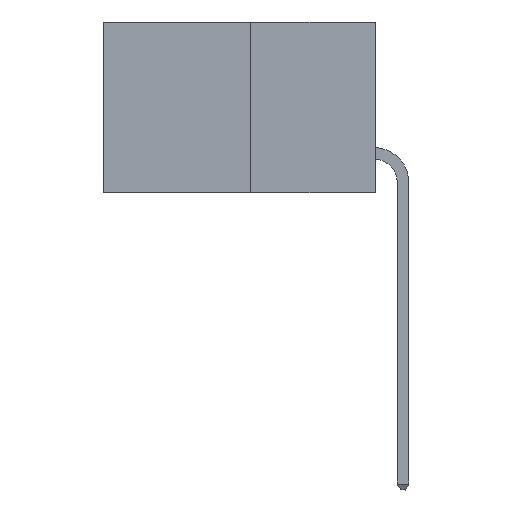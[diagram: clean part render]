
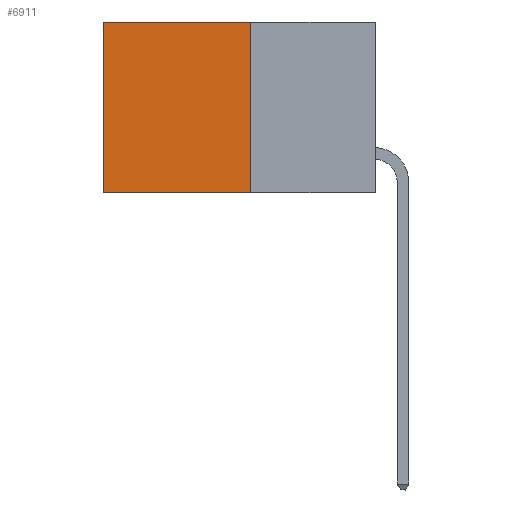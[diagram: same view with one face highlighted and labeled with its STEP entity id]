
A CAD part, left-side view. The second image highlights one B-rep face of the part: STEP entity #6911.
In plain terms, the highlighted planar face has unit normal (-1, 0, 0).
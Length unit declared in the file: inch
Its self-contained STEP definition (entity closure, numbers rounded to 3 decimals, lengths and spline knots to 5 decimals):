
#1206 = VECTOR ( 'NONE', #10832, 39.37008 ) ;
#1775 = VECTOR ( 'NONE', #4129, 39.37008 ) ;
#2823 = LINE ( 'NONE', #6025, #8602 ) ;
#3400 = DIRECTION ( 'NONE',  ( 0., 0., -1. ) ) ;
#4114 = CARTESIAN_POINT ( 'NONE',  ( 0.277, 0.27, 0. ) ) ;
#4129 = DIRECTION ( 'NONE',  ( 0., 1., 0. ) ) ;
#5355 = LINE ( 'NONE', #4114, #1775 ) ;
#5723 = VERTEX_POINT ( 'NONE', #5789 ) ;
#5789 = CARTESIAN_POINT ( 'NONE',  ( 0.277, 0.27, -0.37 ) ) ;
#5966 = CARTESIAN_POINT ( 'NONE',  ( 0.277, 0.59, 0. ) ) ;
#6025 = CARTESIAN_POINT ( 'NONE',  ( 0.277, 0.59, -0.37 ) ) ;
#6221 = CARTESIAN_POINT ( 'NONE',  ( 0.277, 0.27, 0. ) ) ;
#6833 = EDGE_LOOP ( 'NONE', ( #15838, #10210, #9642, #16371 ) ) ;
#6911 = ADVANCED_FACE ( 'NONE', ( #11004 ), #9706, .F. ) ;
#7669 = EDGE_CURVE ( 'NONE', #14370, #8268, #5355, .T. ) ;
#8252 = VERTEX_POINT ( 'NONE', #14915 ) ;
#8268 = VERTEX_POINT ( 'NONE', #5966 ) ;
#8312 = EDGE_CURVE ( 'NONE', #8268, #8252, #2823, .T. ) ;
#8602 = VECTOR ( 'NONE', #3400, 39.37008 ) ;
#9457 = CARTESIAN_POINT ( 'NONE',  ( 0.277, 0.27, -0.37 ) ) ;
#9642 = ORIENTED_EDGE ( 'NONE', *, *, #11752, .F. ) ;
#9647 = DIRECTION ( 'NONE',  ( 0., 0., -1. ) ) ;
#9650 = DIRECTION ( 'NONE',  ( 1., 0., 0. ) ) ;
#9672 = CARTESIAN_POINT ( 'NONE',  ( 0.277, 0.27, -0.37 ) ) ;
#9706 = PLANE ( 'NONE',  #12260 ) ;
#9933 = DIRECTION ( 'NONE',  ( 0., 1., 0. ) ) ;
#10062 = VECTOR ( 'NONE', #9933, 39.37008 ) ;
#10210 = ORIENTED_EDGE ( 'NONE', *, *, #14282, .F. ) ;
#10832 = DIRECTION ( 'NONE',  ( 0., 0., -1. ) ) ;
#11004 = FACE_OUTER_BOUND ( 'NONE', #6833, .T. ) ;
#11752 = EDGE_CURVE ( 'NONE', #14370, #5723, #15129, .T. ) ;
#12260 = AXIS2_PLACEMENT_3D ( 'NONE', #9672, #9650, #9647 ) ;
#13470 = LINE ( 'NONE', #16295, #10062 ) ;
#14282 = EDGE_CURVE ( 'NONE', #5723, #8252, #13470, .T. ) ;
#14370 = VERTEX_POINT ( 'NONE', #6221 ) ;
#14915 = CARTESIAN_POINT ( 'NONE',  ( 0.277, 0.59, -0.37 ) ) ;
#15129 = LINE ( 'NONE', #9457, #1206 ) ;
#15838 = ORIENTED_EDGE ( 'NONE', *, *, #8312, .T. ) ;
#16295 = CARTESIAN_POINT ( 'NONE',  ( 0.277, 0.27, -0.37 ) ) ;
#16371 = ORIENTED_EDGE ( 'NONE', *, *, #7669, .T. ) ;
